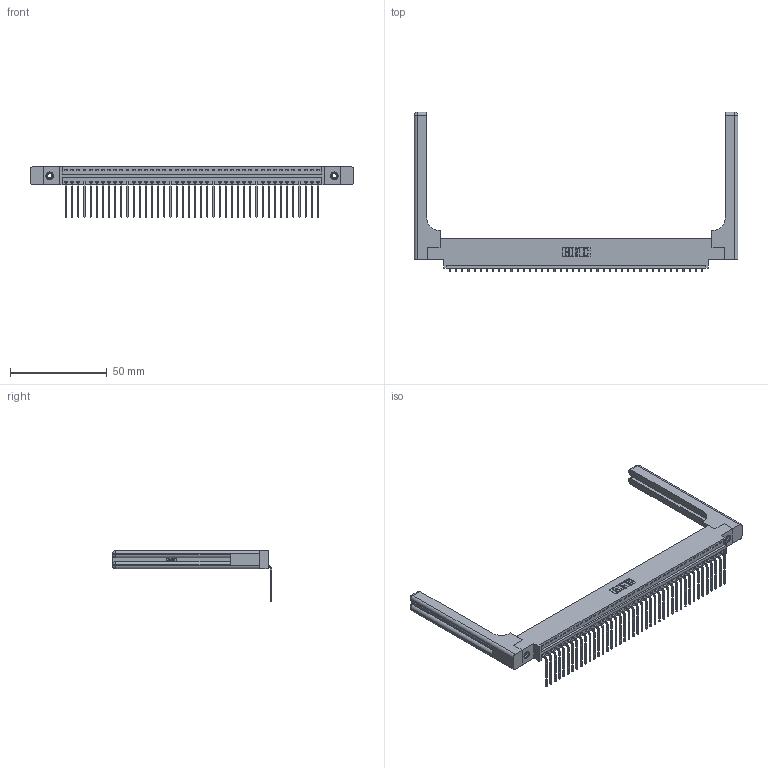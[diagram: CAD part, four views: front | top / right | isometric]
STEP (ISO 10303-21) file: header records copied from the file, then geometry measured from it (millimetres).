
FILE_DESCRIPTION (( 'STEP AP203' ), '1' );
FILE_NAME ('346-042-559-658.STEP', '2022-05-09T15:05:17', ( '' ), ( '' ), 'SwSTEP 2.0', 'SolidWorks 2020', '' );
FILE_SCHEMA (( 'CONFIG_CONTROL_DESIGN' ));
Length unit declared in the file: inch
Products named in the file (5): 345-250-001_345-250-001-102; 345-292-001_558 559 Tail - 1; 346 Part_0.170 Offset - 0.156 Dia-TH; 346-042-559-658; 346-220-058_345-220-058
Assembly tree (47 placements, depth 2):
  346-042-559-658
    346 Part_0.170 Offset - 0.156 Dia-TH
    345-292-001_558 559 Tail - 1  x42
    345-250-001_345-250-001-102  x2
    346-220-058_345-220-058  x2
Bounding box: 167.41 x 82.36 x 26.16 mm (x, y, z)
Volume: 23510.6 mm3; surface area: 26185.2 mm2
Topology: 47 solids, 47 shells, 2916 faces, 8687 edges, 5714 vertices
Faces by surface type: plane 2006, cylinder 850, bspline 36, cone 12, sphere 8, torus 4
Entity records: 31880 total; most frequent: CARTESIAN_POINT 6449, ORIENTED_EDGE 5220, DIRECTION 4618, EDGE_CURVE 2610, VECTOR 2218, LINE 2218, VERTEX_POINT 1730, AXIS2_PLACEMENT_3D 1200
